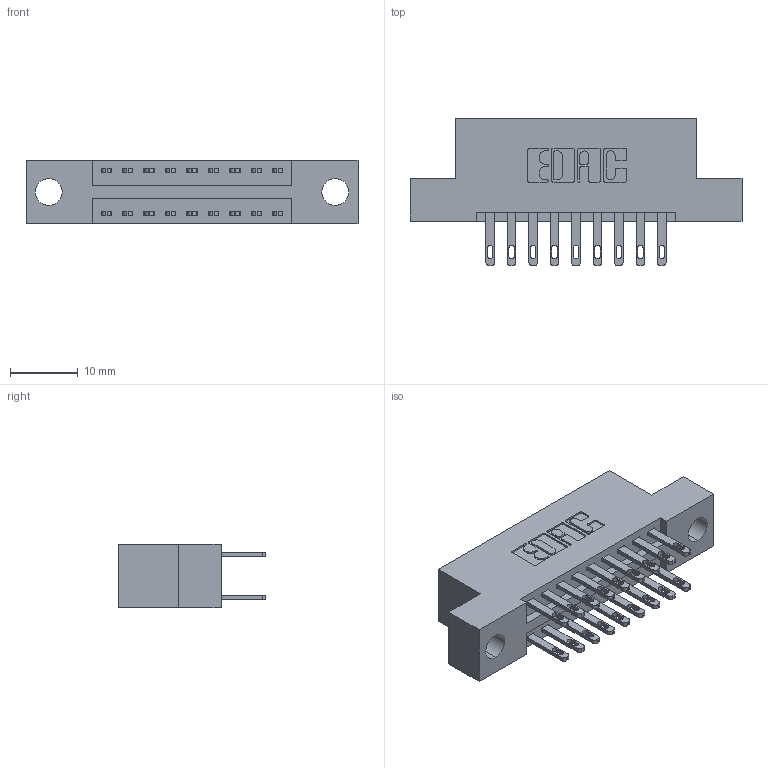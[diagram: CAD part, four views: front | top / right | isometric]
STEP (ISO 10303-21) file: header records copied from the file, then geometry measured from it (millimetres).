
FILE_DESCRIPTION (( 'STEP AP203' ), '1' );
FILE_NAME ('346-018-500-204.STEP', '2022-05-18T16:46:29', ( '' ), ( '' ), 'SwSTEP 2.0', 'SolidWorks 2020', '' );
FILE_SCHEMA (( 'CONFIG_CONTROL_DESIGN' ));
Length unit declared in the file: inch
Products named in the file (3): 346 Part_Flush Mounting Lugs - 0.156 Dia-TH; 345-292-001_345-293-100; 346-018-500-204
Assembly tree (19 placements, depth 2):
  346-018-500-204
    346 Part_Flush Mounting Lugs - 0.156 Dia-TH
    345-292-001_345-293-100  x18
Bounding box: 49.15 x 21.84 x 9.4 mm (x, y, z)
Volume: 4485.4 mm3; surface area: 5683.1 mm2
Topology: 19 solids, 19 shells, 1000 faces, 3011 edges, 2006 vertices
Faces by surface type: plane 612, cylinder 388
Entity records: 10665 total; most frequent: CARTESIAN_POINT 1806, ORIENTED_EDGE 1738, DIRECTION 1645, EDGE_CURVE 869, LINE 697, VECTOR 697, VERTEX_POINT 578, AXIS2_PLACEMENT_3D 474
